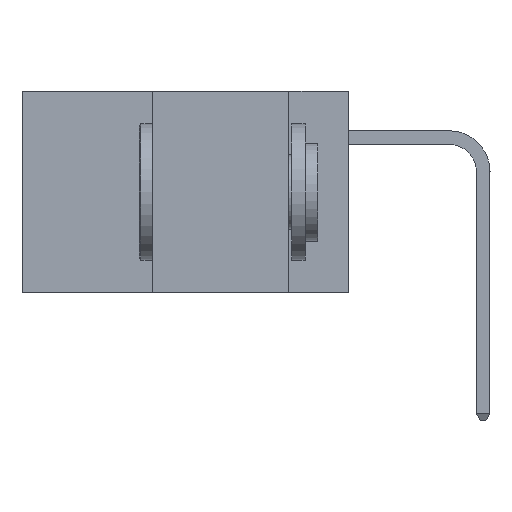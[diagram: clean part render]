
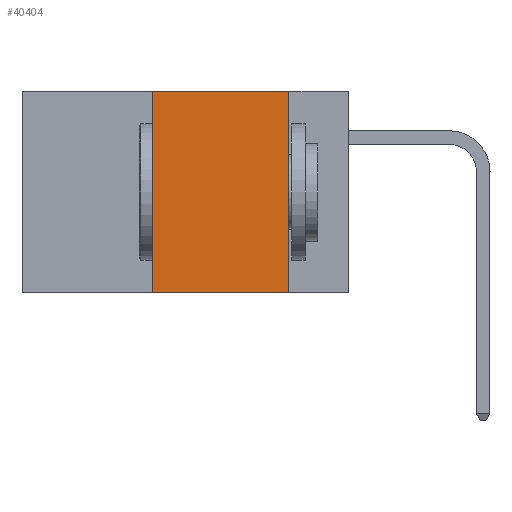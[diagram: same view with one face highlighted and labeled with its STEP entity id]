
A CAD part, left-side view. The second image highlights one B-rep face of the part: STEP entity #40404.
In plain terms, the highlighted planar face has unit normal (-1, 0, 0).
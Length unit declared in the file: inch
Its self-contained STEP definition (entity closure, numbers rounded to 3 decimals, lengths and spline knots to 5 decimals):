
#344 = PLANE ( 'NONE',  #18067 ) ;
#368 = CARTESIAN_POINT ( 'NONE',  ( 0., 0.36, 0. ) ) ;
#725 = CARTESIAN_POINT ( 'NONE',  ( 0., 0.11, 0. ) ) ;
#848 = VECTOR ( 'NONE', #18643, 39.37008 ) ;
#1252 = CARTESIAN_POINT ( 'NONE',  ( 0., 0.36, 0. ) ) ;
#1827 = ORIENTED_EDGE ( 'NONE', *, *, #23197, .F. ) ;
#1961 = LINE ( 'NONE', #16360, #38232 ) ;
#2198 = DIRECTION ( 'NONE',  ( 0., 0., -1. ) ) ;
#2637 = ORIENTED_EDGE ( 'NONE', *, *, #32193, .T. ) ;
#3861 = LINE ( 'NONE', #25973, #34808 ) ;
#5070 = DIRECTION ( 'NONE',  ( 0., -1., 0. ) ) ;
#6311 = EDGE_CURVE ( 'NONE', #10518, #24900, #31827, .T. ) ;
#6682 = CARTESIAN_POINT ( 'NONE',  ( 0., 0.11, -0.37 ) ) ;
#8457 = VECTOR ( 'NONE', #10409, 39.37008 ) ;
#10409 = DIRECTION ( 'NONE',  ( 0., -1., 0. ) ) ;
#10518 = VERTEX_POINT ( 'NONE', #368 ) ;
#12256 = EDGE_LOOP ( 'NONE', ( #42158, #43259, #1827, #2637 ) ) ;
#13833 = VERTEX_POINT ( 'NONE', #38067 ) ;
#16360 = CARTESIAN_POINT ( 'NONE',  ( 0., 0.11, 0. ) ) ;
#16957 = DIRECTION ( 'NONE',  ( 1., 0., 0. ) ) ;
#17271 = DIRECTION ( 'NONE',  ( 0., 0., -1. ) ) ;
#18067 = AXIS2_PLACEMENT_3D ( 'NONE', #24229, #16957, #17271 ) ;
#18163 = LINE ( 'NONE', #1252, #848 ) ;
#18643 = DIRECTION ( 'NONE',  ( 0., 0., 1. ) ) ;
#19534 = FACE_OUTER_BOUND ( 'NONE', #12256, .T. ) ;
#23197 = EDGE_CURVE ( 'NONE', #13833, #10518, #18163, .T. ) ;
#23525 = EDGE_CURVE ( 'NONE', #24900, #39696, #1961, .T. ) ;
#24229 = CARTESIAN_POINT ( 'NONE',  ( 0., 0.6, 0. ) ) ;
#24900 = VERTEX_POINT ( 'NONE', #725 ) ;
#25973 = CARTESIAN_POINT ( 'NONE',  ( 0., 0.6, -0.37 ) ) ;
#31212 = CARTESIAN_POINT ( 'NONE',  ( 0., 0.6, 0. ) ) ;
#31827 = LINE ( 'NONE', #31212, #8457 ) ;
#32193 = EDGE_CURVE ( 'NONE', #13833, #39696, #3861, .T. ) ;
#34808 = VECTOR ( 'NONE', #5070, 39.37008 ) ;
#38067 = CARTESIAN_POINT ( 'NONE',  ( 0., 0.36, -0.37 ) ) ;
#38232 = VECTOR ( 'NONE', #2198, 39.37008 ) ;
#39696 = VERTEX_POINT ( 'NONE', #6682 ) ;
#40404 = ADVANCED_FACE ( 'NONE', ( #19534 ), #344, .F. ) ;
#42158 = ORIENTED_EDGE ( 'NONE', *, *, #23525, .F. ) ;
#43259 = ORIENTED_EDGE ( 'NONE', *, *, #6311, .F. ) ;
